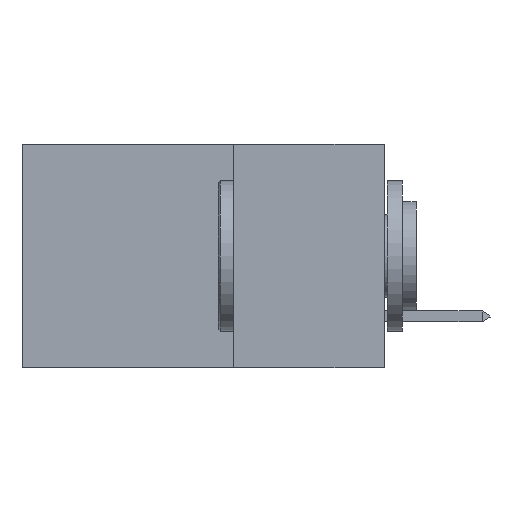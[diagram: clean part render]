
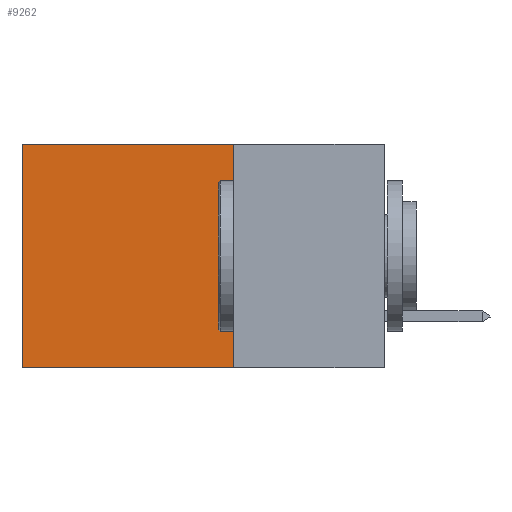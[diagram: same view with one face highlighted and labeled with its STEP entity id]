
A CAD part, left-side view. The second image highlights one B-rep face of the part: STEP entity #9262.
In plain terms, the highlighted planar face has unit normal (-1, 0, 0).
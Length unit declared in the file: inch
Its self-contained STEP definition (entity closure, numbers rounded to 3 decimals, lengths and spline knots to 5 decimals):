
#85 = CARTESIAN_POINT ( 'NONE',  ( 0.2875, 0.25, 0. ) ) ;
#2998 = EDGE_CURVE ( 'NONE', #25104, #8267, #24882, .T. ) ;
#4028 = ORIENTED_EDGE ( 'NONE', *, *, #44904, .F. ) ;
#4740 = VERTEX_POINT ( 'NONE', #10586 ) ;
#5501 = ORIENTED_EDGE ( 'NONE', *, *, #14055, .T. ) ;
#6024 = VERTEX_POINT ( 'NONE', #85 ) ;
#6174 = ORIENTED_EDGE ( 'NONE', *, *, #2998, .T. ) ;
#8267 = VERTEX_POINT ( 'NONE', #40004 ) ;
#8803 = CARTESIAN_POINT ( 'NONE',  ( 0.2875, 0.25, -0.37 ) ) ;
#9262 = ADVANCED_FACE ( 'NONE', ( #47575 ), #15731, .F. ) ;
#10586 = CARTESIAN_POINT ( 'NONE',  ( 0.2875, 0.25, -0.37 ) ) ;
#11094 = EDGE_LOOP ( 'NONE', ( #6174, #4028, #28026, #5501 ) ) ;
#13350 = CARTESIAN_POINT ( 'NONE',  ( 0.2875, 0.25, 0. ) ) ;
#14055 = EDGE_CURVE ( 'NONE', #6024, #25104, #37232, .T. ) ;
#15731 = PLANE ( 'NONE',  #44867 ) ;
#21803 = DIRECTION ( 'NONE',  ( 0., 1., 0. ) ) ;
#22336 = CARTESIAN_POINT ( 'NONE',  ( 0.2875, 0.25, 0. ) ) ;
#22455 = LINE ( 'NONE', #13350, #44027 ) ;
#23125 = LINE ( 'NONE', #8803, #41801 ) ;
#24197 = CARTESIAN_POINT ( 'NONE',  ( 0.2875, 0.6, 0. ) ) ;
#24882 = LINE ( 'NONE', #24197, #29585 ) ;
#25104 = VERTEX_POINT ( 'NONE', #30717 ) ;
#28026 = ORIENTED_EDGE ( 'NONE', *, *, #37098, .F. ) ;
#29585 = VECTOR ( 'NONE', #43098, 39.37008 ) ;
#30717 = CARTESIAN_POINT ( 'NONE',  ( 0.2875, 0.6, 0. ) ) ;
#31065 = DIRECTION ( 'NONE',  ( 1., 0., 0. ) ) ;
#31395 = VECTOR ( 'NONE', #21803, 39.37008 ) ;
#37098 = EDGE_CURVE ( 'NONE', #6024, #4740, #22455, .T. ) ;
#37232 = LINE ( 'NONE', #22336, #31395 ) ;
#38076 = DIRECTION ( 'NONE',  ( 0., 0., -1. ) ) ;
#39475 = DIRECTION ( 'NONE',  ( 0., 0., -1. ) ) ;
#40004 = CARTESIAN_POINT ( 'NONE',  ( 0.2875, 0.6, -0.37 ) ) ;
#41801 = VECTOR ( 'NONE', #45701, 39.37008 ) ;
#42140 = CARTESIAN_POINT ( 'NONE',  ( 0.2875, 0.25, 0. ) ) ;
#43098 = DIRECTION ( 'NONE',  ( 0., 0., -1. ) ) ;
#44027 = VECTOR ( 'NONE', #39475, 39.37008 ) ;
#44867 = AXIS2_PLACEMENT_3D ( 'NONE', #42140, #31065, #38076 ) ;
#44904 = EDGE_CURVE ( 'NONE', #4740, #8267, #23125, .T. ) ;
#45701 = DIRECTION ( 'NONE',  ( 0., 1., 0. ) ) ;
#47575 = FACE_OUTER_BOUND ( 'NONE', #11094, .T. ) ;
